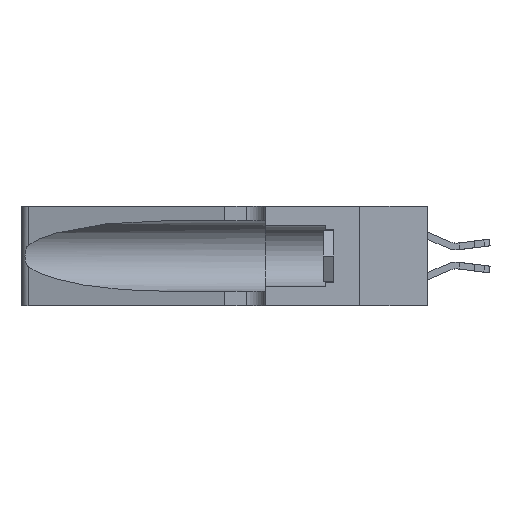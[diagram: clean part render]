
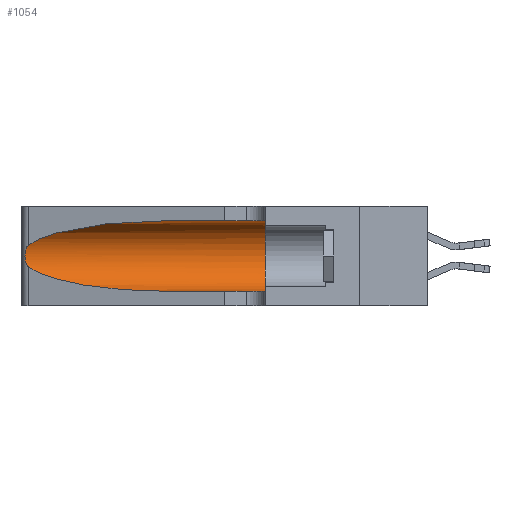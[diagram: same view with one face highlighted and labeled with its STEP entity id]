
A CAD part, left-side view. The second image highlights one B-rep face of the part: STEP entity #1054.
In plain terms, the highlighted cylindrical face has radius 3.308 mm (diameter 6.617 mm), a partial arc.
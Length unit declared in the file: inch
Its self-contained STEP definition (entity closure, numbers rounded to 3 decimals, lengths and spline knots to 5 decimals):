
#41 = CARTESIAN_POINT ( 'NONE',  ( 0.1305, 1.61858, 0.31525 ) ) ;
#821 = AXIS2_PLACEMENT_3D ( 'NONE', #8781, #8646, #8698 ) ;
#1054 = ADVANCED_FACE ( 'NONE', ( #3524 ), #20353, .F. ) ;
#1384 = ORIENTED_EDGE ( 'NONE', *, *, #11641, .F. ) ;
#1589 = CARTESIAN_POINT ( 'NONE',  ( 0.18966, 0.96281, 0.31525 ) ) ;
#1820 = CARTESIAN_POINT ( 'NONE',  ( 0.25789, 1.23486, 0.15765 ) ) ;
#2979 = VECTOR ( 'NONE', #18775, 39.37008 ) ;
#3277 = CARTESIAN_POINT ( 'NONE',  ( 0.1305, 1.61858, 0.05475 ) ) ;
#3524 = FACE_OUTER_BOUND ( 'NONE', #5669, .T. ) ;
#3981 = CARTESIAN_POINT ( 'NONE',  ( 0.25555, 1.22994, 0.2215 ) ) ;
#4080 = CARTESIAN_POINT ( 'NONE',  ( 0.25555, 1.22993, 0.14849 ) ) ;
#5077 = VERTEX_POINT ( 'NONE', #8606 ) ;
#5669 = EDGE_LOOP ( 'NONE', ( #21998, #22668, #5953, #11848, #23962, #1384 ) ) ;
#5953 = ORIENTED_EDGE ( 'NONE', *, *, #27626, .T. ) ;
#6029 = VERTEX_POINT ( 'NONE', #8260 ) ;
#6150 = CIRCLE ( 'NONE', #20118, 0.13025 ) ;
#6425 = CARTESIAN_POINT ( 'NONE',  ( 0.25487, 1.22718, 0.14631 ) ) ;
#6728 = DIRECTION ( 'NONE',  ( 0., 1., 0. ) ) ;
#7929 = VERTEX_POINT ( 'NONE', #16419 ) ;
#8260 = CARTESIAN_POINT ( 'NONE',  ( 0.25487, 1.22718, 0.22369 ) ) ;
#8344 = CARTESIAN_POINT ( 'NONE',  ( 0.2373, 1.15595, 0.28018 ) ) ;
#8476 = CARTESIAN_POINT ( 'NONE',  ( 0.25787, 1.23484, 0.2124 ) ) ;
#8606 = CARTESIAN_POINT ( 'NONE',  ( 0.1305, 0.72297, 0.05475 ) ) ;
#8642 =( BOUNDED_CURVE ( )  B_SPLINE_CURVE ( 3, ( #17065, #1589, #8344, #23507 ),
 .UNSPECIFIED., .F., .T. ) 
 B_SPLINE_CURVE_WITH_KNOTS ( ( 4, 4 ),
 ( 1.5708, 2.84003 ),
 .UNSPECIFIED. ) 
 CURVE ( )  GEOMETRIC_REPRESENTATION_ITEM ( )  RATIONAL_B_SPLINE_CURVE ( ( 1., 0.87, 0.87, 1. ) ) 
 REPRESENTATION_ITEM ( '' )  );
#8646 = DIRECTION ( 'NONE',  ( 0., -1., 0. ) ) ;
#8649 = CARTESIAN_POINT ( 'NONE',  ( 0.2373, 1.15595, 0.08982 ) ) ;
#8698 = DIRECTION ( 'NONE',  ( 0., 0., -1. ) ) ;
#8781 = CARTESIAN_POINT ( 'NONE',  ( 0.1305, 1.61858, 0.185 ) ) ;
#8892 = LINE ( 'NONE', #3277, #2979 ) ;
#10693 = CARTESIAN_POINT ( 'NONE',  ( 0.26018, 1.23835, 0.19895 ) ) ;
#11641 = EDGE_CURVE ( 'NONE', #7929, #24183, #23235, .T. ) ;
#11848 = ORIENTED_EDGE ( 'NONE', *, *, #13106, .T. ) ;
#12778 = EDGE_CURVE ( 'NONE', #24183, #25889, #6150, .T. ) ;
#12906 = CARTESIAN_POINT ( 'NONE',  ( 0.26075, 1.23896, 0.178 ) ) ;
#13106 = EDGE_CURVE ( 'NONE', #5077, #25889, #8892, .T. ) ;
#15000 = CARTESIAN_POINT ( 'NONE',  ( 0.25487, 1.22718, 0.22369 ) ) ;
#15104 = CARTESIAN_POINT ( 'NONE',  ( 0.25856, 1.23593, 0.16098 ) ) ;
#15283 = CARTESIAN_POINT ( 'NONE',  ( 0.1305, 0.72297, 0.05475 ) ) ;
#16419 = CARTESIAN_POINT ( 'NONE',  ( 0.1305, 0.72297, 0.31525 ) ) ;
#17065 = CARTESIAN_POINT ( 'NONE',  ( 0.1305, 0.72297, 0.31525 ) ) ;
#17290 = CARTESIAN_POINT ( 'NONE',  ( 0.25639, 1.23186, 0.15144 ) ) ;
#17555 = VECTOR ( 'NONE', #17793, 39.37008 ) ;
#17793 = DIRECTION ( 'NONE',  ( 0., -1., 0. ) ) ;
#18775 = DIRECTION ( 'NONE',  ( 0., -1., 0. ) ) ;
#19459 = CARTESIAN_POINT ( 'NONE',  ( 0.25487, 1.22718, 0.14631 ) ) ;
#19770 = VERTEX_POINT ( 'NONE', #23159 ) ;
#19822 = CARTESIAN_POINT ( 'NONE',  ( 0.1305, 0.35, 0.185 ) ) ;
#20118 = AXIS2_PLACEMENT_3D ( 'NONE', #19822, #6728, #21954 ) ;
#20353 = CYLINDRICAL_SURFACE ( 'NONE', #821, 0.13025 ) ;
#20364 = EDGE_CURVE ( 'NONE', #6029, #19770, #23729, .T. ) ;
#21503 = CARTESIAN_POINT ( 'NONE',  ( 0.25639, 1.23184, 0.21858 ) ) ;
#21954 = DIRECTION ( 'NONE',  ( 0., 0., 1. ) ) ;
#21998 = ORIENTED_EDGE ( 'NONE', *, *, #23726, .T. ) ;
#22216 = CARTESIAN_POINT ( 'NONE',  ( 0.1305, 0.35, 0.05475 ) ) ;
#22668 = ORIENTED_EDGE ( 'NONE', *, *, #20364, .T. ) ;
#23159 = CARTESIAN_POINT ( 'NONE',  ( 0.25487, 1.22718, 0.14631 ) ) ;
#23235 = LINE ( 'NONE', #41, #17555 ) ;
#23507 = CARTESIAN_POINT ( 'NONE',  ( 0.25487, 1.22718, 0.22369 ) ) ;
#23624 = CARTESIAN_POINT ( 'NONE',  ( 0.25854, 1.2359, 0.20912 ) ) ;
#23726 = EDGE_CURVE ( 'NONE', #7929, #6029, #8642, .T. ) ;
#23729 = B_SPLINE_CURVE_WITH_KNOTS ( 'NONE', 3,
 ( #15000, #3981, #21503, #8476, #23624, #10693, #25779, #12906, #27917, #15104, #1820, #17290, #4080, #19459 ),
 .UNSPECIFIED., .F., .F.,
 ( 4, 2, 2, 2, 2, 2, 4 ),
 ( 0., 0.00027, 0.00053, 0.00107, 0.0016, 0.00187, 0.00214 ),
 .UNSPECIFIED. ) ;
#23962 = ORIENTED_EDGE ( 'NONE', *, *, #12778, .F. ) ;
#24183 = VERTEX_POINT ( 'NONE', #24887 ) ;
#24887 = CARTESIAN_POINT ( 'NONE',  ( 0.1305, 0.35, 0.31525 ) ) ;
#25779 = CARTESIAN_POINT ( 'NONE',  ( 0.26075, 1.23896, 0.19203 ) ) ;
#25889 = VERTEX_POINT ( 'NONE', #22216 ) ;
#26652 =( BOUNDED_CURVE ( )  B_SPLINE_CURVE ( 3, ( #6425, #8649, #28082, #15283 ),
 .UNSPECIFIED., .F., .T. ) 
 B_SPLINE_CURVE_WITH_KNOTS ( ( 4, 4 ),
 ( 3.44316, 4.71239 ),
 .UNSPECIFIED. ) 
 CURVE ( )  GEOMETRIC_REPRESENTATION_ITEM ( )  RATIONAL_B_SPLINE_CURVE ( ( 1., 0.87, 0.87, 1. ) ) 
 REPRESENTATION_ITEM ( '' )  );
#27626 = EDGE_CURVE ( 'NONE', #19770, #5077, #26652, .T. ) ;
#27917 = CARTESIAN_POINT ( 'NONE',  ( 0.26017, 1.23833, 0.17102 ) ) ;
#28082 = CARTESIAN_POINT ( 'NONE',  ( 0.18966, 0.96281, 0.05475 ) ) ;
